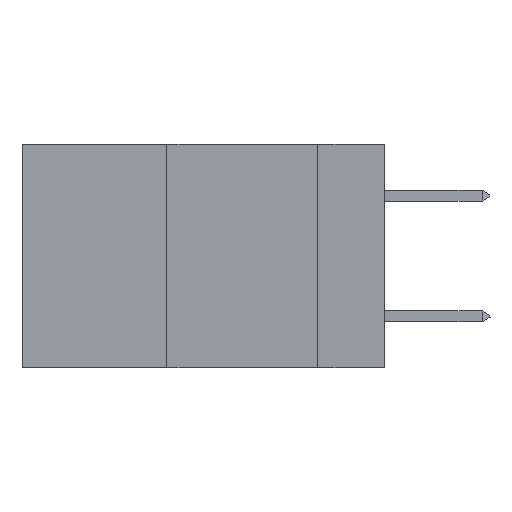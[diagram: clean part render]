
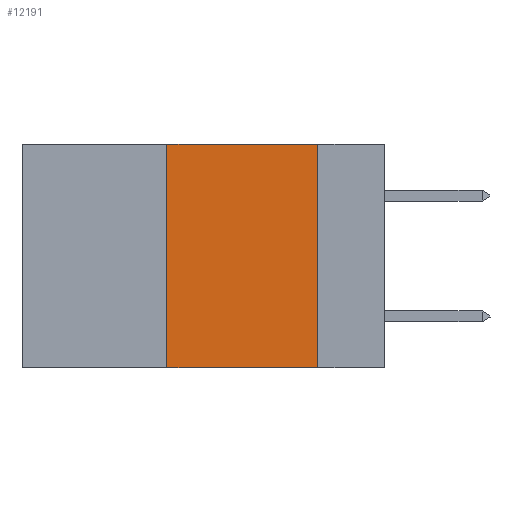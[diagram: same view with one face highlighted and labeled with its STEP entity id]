
A CAD part, left-side view. The second image highlights one B-rep face of the part: STEP entity #12191.
In plain terms, the highlighted planar face has unit normal (-1, 0, 0).
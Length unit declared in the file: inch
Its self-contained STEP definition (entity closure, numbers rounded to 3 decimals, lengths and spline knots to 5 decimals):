
#58 = CARTESIAN_POINT ( 'NONE',  ( 0., 0.36, 0. ) ) ;
#203 = EDGE_CURVE ( 'NONE', #6092, #18845, #17317, .T. ) ;
#367 = CARTESIAN_POINT ( 'NONE',  ( 0., 0.6, 0. ) ) ;
#669 = VECTOR ( 'NONE', #11541, 39.37008 ) ;
#1342 = CARTESIAN_POINT ( 'NONE',  ( 0., 0.6, -0.37 ) ) ;
#4557 = FACE_OUTER_BOUND ( 'NONE', #21345, .T. ) ;
#5622 = EDGE_CURVE ( 'NONE', #6092, #12308, #6075, .T. ) ;
#6075 = LINE ( 'NONE', #58, #18517 ) ;
#6092 = VERTEX_POINT ( 'NONE', #13085 ) ;
#7005 = DIRECTION ( 'NONE',  ( 0., 0., -1. ) ) ;
#8024 = LINE ( 'NONE', #11565, #24383 ) ;
#9450 = LINE ( 'NONE', #15469, #669 ) ;
#9643 = EDGE_CURVE ( 'NONE', #12308, #16446, #8024, .T. ) ;
#11541 = DIRECTION ( 'NONE',  ( 0., 0., -1. ) ) ;
#11565 = CARTESIAN_POINT ( 'NONE',  ( 0., 0.6, 0. ) ) ;
#11647 = ORIENTED_EDGE ( 'NONE', *, *, #9643, .F. ) ;
#12191 = ADVANCED_FACE ( 'NONE', ( #4557 ), #16962, .F. ) ;
#12308 = VERTEX_POINT ( 'NONE', #19688 ) ;
#12582 = VECTOR ( 'NONE', #14837, 39.37008 ) ;
#13085 = CARTESIAN_POINT ( 'NONE',  ( 0., 0.36, -0.37 ) ) ;
#14058 = DIRECTION ( 'NONE',  ( 0., -1., 0. ) ) ;
#14837 = DIRECTION ( 'NONE',  ( 0., -1., 0. ) ) ;
#15469 = CARTESIAN_POINT ( 'NONE',  ( 0., 0.11, 0. ) ) ;
#16095 = DIRECTION ( 'NONE',  ( 1., 0., 0. ) ) ;
#16446 = VERTEX_POINT ( 'NONE', #20343 ) ;
#16962 = PLANE ( 'NONE',  #18438 ) ;
#17317 = LINE ( 'NONE', #1342, #12582 ) ;
#17462 = CARTESIAN_POINT ( 'NONE',  ( 0., 0.11, -0.37 ) ) ;
#17623 = ORIENTED_EDGE ( 'NONE', *, *, #5622, .F. ) ;
#18438 = AXIS2_PLACEMENT_3D ( 'NONE', #367, #16095, #7005 ) ;
#18517 = VECTOR ( 'NONE', #20209, 39.37008 ) ;
#18845 = VERTEX_POINT ( 'NONE', #17462 ) ;
#18991 = ORIENTED_EDGE ( 'NONE', *, *, #203, .T. ) ;
#19665 = ORIENTED_EDGE ( 'NONE', *, *, #20677, .F. ) ;
#19688 = CARTESIAN_POINT ( 'NONE',  ( 0., 0.36, 0. ) ) ;
#20209 = DIRECTION ( 'NONE',  ( 0., 0., 1. ) ) ;
#20343 = CARTESIAN_POINT ( 'NONE',  ( 0., 0.11, 0. ) ) ;
#20677 = EDGE_CURVE ( 'NONE', #16446, #18845, #9450, .T. ) ;
#21345 = EDGE_LOOP ( 'NONE', ( #19665, #11647, #17623, #18991 ) ) ;
#24383 = VECTOR ( 'NONE', #14058, 39.37008 ) ;
